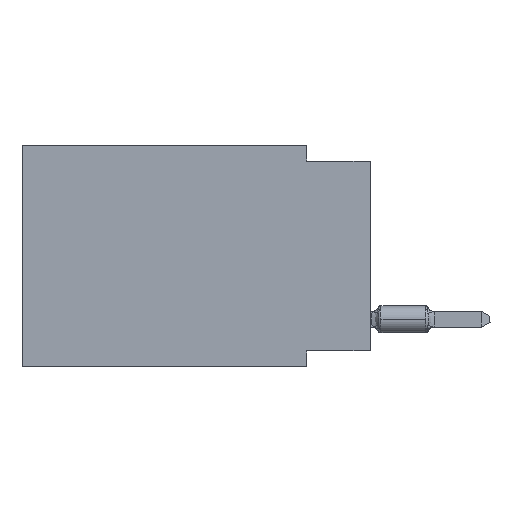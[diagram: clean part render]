
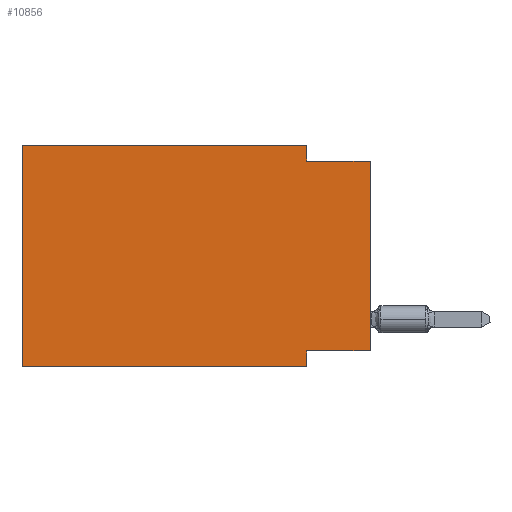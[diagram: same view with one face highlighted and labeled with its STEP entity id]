
A CAD part, left-side view. The second image highlights one B-rep face of the part: STEP entity #10856.
In plain terms, the highlighted planar face has unit normal (-1, 0, 0).
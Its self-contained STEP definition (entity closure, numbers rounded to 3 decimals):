
#469 = LINE ( 'NONE', #16393, #22081 ) ;
#675 = VERTEX_POINT ( 'NONE', #13039 ) ;
#937 = DIRECTION ( 'NONE',  ( 0., 0., -1. ) ) ;
#1064 = DIRECTION ( 'NONE',  ( 1., 0., 0. ) ) ;
#1068 = VECTOR ( 'NONE', #9612, 1000. ) ;
#1393 = CARTESIAN_POINT ( 'NONE',  ( 0., 2.54, 0. ) ) ;
#1523 = CARTESIAN_POINT ( 'NONE',  ( 0., 13.97, -8.89 ) ) ;
#1767 = ORIENTED_EDGE ( 'NONE', *, *, #24436, .F. ) ;
#2319 = ORIENTED_EDGE ( 'NONE', *, *, #5359, .F. ) ;
#2787 = CARTESIAN_POINT ( 'NONE',  ( 0., 13.97, 0. ) ) ;
#3197 = LINE ( 'NONE', #11182, #1068 ) ;
#3654 = CARTESIAN_POINT ( 'NONE',  ( 0., 0., -0.635 ) ) ;
#4381 = VERTEX_POINT ( 'NONE', #20812 ) ;
#4497 = DIRECTION ( 'NONE',  ( 0., 0., 1. ) ) ;
#5327 = CARTESIAN_POINT ( 'NONE',  ( 0., 13.97, -8.89 ) ) ;
#5359 = EDGE_CURVE ( 'NONE', #4381, #675, #3197, .T. ) ;
#6008 = LINE ( 'NONE', #7975, #25456 ) ;
#6176 = VECTOR ( 'NONE', #9088, 1000. ) ;
#7591 = EDGE_CURVE ( 'NONE', #675, #18628, #8956, .T. ) ;
#7975 = CARTESIAN_POINT ( 'NONE',  ( 0., 13.97, 0. ) ) ;
#8956 = LINE ( 'NONE', #24995, #6176 ) ;
#9088 = DIRECTION ( 'NONE',  ( 0., 0., -1. ) ) ;
#9566 = DIRECTION ( 'NONE',  ( 0., -1., 0. ) ) ;
#9612 = DIRECTION ( 'NONE',  ( 0., 1., 0. ) ) ;
#9625 = ORIENTED_EDGE ( 'NONE', *, *, #19033, .F. ) ;
#9835 = ORIENTED_EDGE ( 'NONE', *, *, #17991, .F. ) ;
#10856 = ADVANCED_FACE ( 'NONE', ( #20794 ), #23126, .F. ) ;
#11182 = CARTESIAN_POINT ( 'NONE',  ( 0., 0., -8.255 ) ) ;
#11216 = LINE ( 'NONE', #5327, #19173 ) ;
#11476 = EDGE_CURVE ( 'NONE', #16293, #23903, #24480, .T. ) ;
#11628 = ORIENTED_EDGE ( 'NONE', *, *, #22864, .T. ) ;
#11991 = EDGE_LOOP ( 'NONE', ( #11628, #9625, #13212, #1767, #9835, #23654, #21752, #2319 ) ) ;
#13039 = CARTESIAN_POINT ( 'NONE',  ( 0., 2.54, -8.255 ) ) ;
#13212 = ORIENTED_EDGE ( 'NONE', *, *, #11476, .F. ) ;
#13709 = LINE ( 'NONE', #3654, #16881 ) ;
#13870 = VERTEX_POINT ( 'NONE', #1523 ) ;
#14128 = CARTESIAN_POINT ( 'NONE',  ( 0., 13.97, 0. ) ) ;
#14171 = CARTESIAN_POINT ( 'NONE',  ( 0., 2.54, -0.635 ) ) ;
#14268 = LINE ( 'NONE', #2787, #20420 ) ;
#14506 = CARTESIAN_POINT ( 'NONE',  ( 0., 0., -0.635 ) ) ;
#14720 = AXIS2_PLACEMENT_3D ( 'NONE', #16608, #1064, #937 ) ;
#15586 = CARTESIAN_POINT ( 'NONE',  ( 0., 2.54, -8.89 ) ) ;
#16293 = VERTEX_POINT ( 'NONE', #1393 ) ;
#16380 = CARTESIAN_POINT ( 'NONE',  ( 0., 2.54, 0. ) ) ;
#16393 = CARTESIAN_POINT ( 'NONE',  ( 0., 0., 0. ) ) ;
#16608 = CARTESIAN_POINT ( 'NONE',  ( 0., 13.97, 0. ) ) ;
#16881 = VECTOR ( 'NONE', #9566, 1000. ) ;
#17606 = VERTEX_POINT ( 'NONE', #14506 ) ;
#17991 = EDGE_CURVE ( 'NONE', #13870, #21543, #6008, .T. ) ;
#18628 = VERTEX_POINT ( 'NONE', #15586 ) ;
#18713 = DIRECTION ( 'NONE',  ( 0., -1., 0. ) ) ;
#19033 = EDGE_CURVE ( 'NONE', #23903, #17606, #13709, .T. ) ;
#19173 = VECTOR ( 'NONE', #23083, 1000. ) ;
#20420 = VECTOR ( 'NONE', #18713, 1000. ) ;
#20794 = FACE_OUTER_BOUND ( 'NONE', #11991, .T. ) ;
#20812 = CARTESIAN_POINT ( 'NONE',  ( 0., 0., -8.255 ) ) ;
#21431 = VECTOR ( 'NONE', #24611, 1000. ) ;
#21543 = VERTEX_POINT ( 'NONE', #14128 ) ;
#21752 = ORIENTED_EDGE ( 'NONE', *, *, #7591, .F. ) ;
#22081 = VECTOR ( 'NONE', #4497, 1000. ) ;
#22508 = EDGE_CURVE ( 'NONE', #13870, #18628, #11216, .T. ) ;
#22864 = EDGE_CURVE ( 'NONE', #4381, #17606, #469, .T. ) ;
#23083 = DIRECTION ( 'NONE',  ( 0., -1., 0. ) ) ;
#23126 = PLANE ( 'NONE',  #14720 ) ;
#23654 = ORIENTED_EDGE ( 'NONE', *, *, #22508, .T. ) ;
#23903 = VERTEX_POINT ( 'NONE', #14171 ) ;
#24158 = DIRECTION ( 'NONE',  ( 0., 0., 1. ) ) ;
#24436 = EDGE_CURVE ( 'NONE', #21543, #16293, #14268, .T. ) ;
#24480 = LINE ( 'NONE', #16380, #21431 ) ;
#24611 = DIRECTION ( 'NONE',  ( 0., 0., -1. ) ) ;
#24995 = CARTESIAN_POINT ( 'NONE',  ( 0., 2.54, -8.89 ) ) ;
#25456 = VECTOR ( 'NONE', #24158, 1000. ) ;
